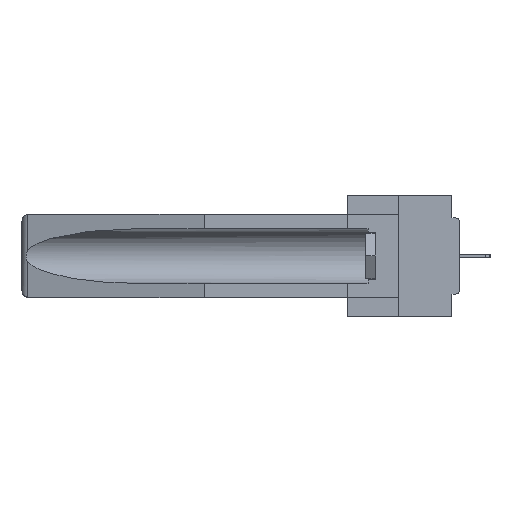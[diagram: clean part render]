
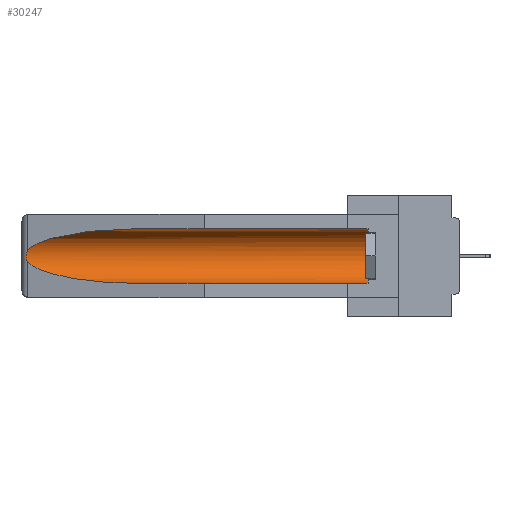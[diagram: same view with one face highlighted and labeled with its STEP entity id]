
A CAD part, left-side view. The second image highlights one B-rep face of the part: STEP entity #30247.
In plain terms, the highlighted cylindrical face has radius 2.857 mm (diameter 5.715 mm), a partial arc.
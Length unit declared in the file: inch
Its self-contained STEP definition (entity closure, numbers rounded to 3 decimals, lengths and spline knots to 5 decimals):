
#1117 = FACE_OUTER_BOUND ( 'NONE', #20640, .T. ) ;
#1626 = LINE ( 'NONE', #13462, #16823 ) ;
#1661 = CARTESIAN_POINT ( 'NONE',  ( 0.155, 1.07973, -0.284 ) ) ;
#2852 = CARTESIAN_POINT ( 'NONE',  ( 0.26597, 1.52961, -0.15275 ) ) ;
#3808 = EDGE_CURVE ( 'NONE', #28295, #29521, #8034, .T. ) ;
#3958 = ORIENTED_EDGE ( 'NONE', *, *, #11584, .T. ) ;
#4054 = CARTESIAN_POINT ( 'NONE',  ( 0.155, 0.126, -0.1715 ) ) ;
#4344 = VERTEX_POINT ( 'NONE', #22778 ) ;
#4686 = CARTESIAN_POINT ( 'NONE',  ( 0.155, 1.07973, -0.059 ) ) ;
#5570 = EDGE_CURVE ( 'NONE', #17161, #17601, #1626, .T. ) ;
#6491 = ORIENTED_EDGE ( 'NONE', *, *, #11716, .F. ) ;
#6703 = VECTOR ( 'NONE', #26251, 39.37008 ) ;
#6877 = CARTESIAN_POINT ( 'NONE',  ( 0.26537, 1.52718, -0.19328 ) ) ;
#7277 =( BOUNDED_CURVE ( )  B_SPLINE_CURVE ( 3, ( #10689, #28624, #8088, #26341 ),
 .UNSPECIFIED., .F., .F. ) 
 B_SPLINE_CURVE_WITH_KNOTS ( ( 4, 4 ),
 ( 0.1948, 1.5708 ),
 .UNSPECIFIED. ) 
 CURVE ( )  GEOMETRIC_REPRESENTATION_ITEM ( )  RATIONAL_B_SPLINE_CURVE ( ( 1., 0.848, 0.848, 1. ) ) 
 REPRESENTATION_ITEM ( '' )  );
#8034 = B_SPLINE_CURVE_WITH_KNOTS ( 'NONE', 3,
 ( #14870, #2852, #12246, #28824, #15017, #26208, #19475, #16701, #21770, #21601 ),
 .UNSPECIFIED., .F., .F.,
 ( 4, 2, 2, 2, 4 ),
 ( 0., 0.00029, 0.00058, 0.00087, 0.00117 ),
 .UNSPECIFIED. ) ;
#8057 = DIRECTION ( 'NONE',  ( 0., 1., 0. ) ) ;
#8088 = CARTESIAN_POINT ( 'NONE',  ( 0.21114, 1.30732, -0.284 ) ) ;
#10439 = EDGE_CURVE ( 'NONE', #29521, #12492, #7277, .T. ) ;
#10689 = CARTESIAN_POINT ( 'NONE',  ( 0.26537, 1.52718, -0.19328 ) ) ;
#10832 = DIRECTION ( 'NONE',  ( 0., -1., 0. ) ) ;
#11584 = EDGE_CURVE ( 'NONE', #4344, #17161, #13330, .T. ) ;
#11716 = EDGE_CURVE ( 'NONE', #4344, #12492, #23651, .T. ) ;
#12151 = ORIENTED_EDGE ( 'NONE', *, *, #10439, .T. ) ;
#12246 = CARTESIAN_POINT ( 'NONE',  ( 0.26654, 1.53092, -0.15636 ) ) ;
#12492 = VERTEX_POINT ( 'NONE', #1661 ) ;
#13330 = CIRCLE ( 'NONE', #18687, 0.1125 ) ;
#13462 = CARTESIAN_POINT ( 'NONE',  ( 0.155, -0.30754, -0.059 ) ) ;
#14870 = CARTESIAN_POINT ( 'NONE',  ( 0.26537, 1.52718, -0.14972 ) ) ;
#15017 = CARTESIAN_POINT ( 'NONE',  ( 0.2675, 1.53308, -0.16763 ) ) ;
#15663 = CARTESIAN_POINT ( 'NONE',  ( 0.26537, 1.52718, -0.14972 ) ) ;
#15746 = DIRECTION ( 'NONE',  ( 0., 0., 1. ) ) ;
#16701 = CARTESIAN_POINT ( 'NONE',  ( 0.26655, 1.53094, -0.18657 ) ) ;
#16823 = VECTOR ( 'NONE', #22351, 39.37008 ) ;
#17161 = VERTEX_POINT ( 'NONE', #27522 ) ;
#17254 = DIRECTION ( 'NONE',  ( 0., 0., 1. ) ) ;
#17601 = VERTEX_POINT ( 'NONE', #4686 ) ;
#18124 = CARTESIAN_POINT ( 'NONE',  ( 0.21114, 1.30732, -0.059 ) ) ;
#18189 = ORIENTED_EDGE ( 'NONE', *, *, #20314, .T. ) ;
#18687 = AXIS2_PLACEMENT_3D ( 'NONE', #4054, #10832, #15746 ) ;
#19475 = CARTESIAN_POINT ( 'NONE',  ( 0.2673, 1.53269, -0.17917 ) ) ;
#19799 = ORIENTED_EDGE ( 'NONE', *, *, #5570, .T. ) ;
#20237 = CARTESIAN_POINT ( 'NONE',  ( 0.26537, 1.52718, -0.14972 ) ) ;
#20314 = EDGE_CURVE ( 'NONE', #17601, #28295, #28079, .T. ) ;
#20640 = EDGE_LOOP ( 'NONE', ( #18189, #26591, #12151, #6491, #3958, #19799 ) ) ;
#21081 = AXIS2_PLACEMENT_3D ( 'NONE', #21692, #8057, #17254 ) ;
#21601 = CARTESIAN_POINT ( 'NONE',  ( 0.26537, 1.52718, -0.19328 ) ) ;
#21692 = CARTESIAN_POINT ( 'NONE',  ( 0.155, -0.30754, -0.1715 ) ) ;
#21770 = CARTESIAN_POINT ( 'NONE',  ( 0.26597, 1.5296, -0.19026 ) ) ;
#22351 = DIRECTION ( 'NONE',  ( 0., 1., 0. ) ) ;
#22778 = CARTESIAN_POINT ( 'NONE',  ( 0.155, 0.126, -0.284 ) ) ;
#23651 = LINE ( 'NONE', #26092, #6703 ) ;
#24632 = CYLINDRICAL_SURFACE ( 'NONE', #21081, 0.1125 ) ;
#26092 = CARTESIAN_POINT ( 'NONE',  ( 0.155, -0.30754, -0.284 ) ) ;
#26208 = CARTESIAN_POINT ( 'NONE',  ( 0.2675, 1.53308, -0.17534 ) ) ;
#26251 = DIRECTION ( 'NONE',  ( 0., 1., 0. ) ) ;
#26341 = CARTESIAN_POINT ( 'NONE',  ( 0.155, 1.07973, -0.284 ) ) ;
#26591 = ORIENTED_EDGE ( 'NONE', *, *, #3808, .T. ) ;
#27332 = CARTESIAN_POINT ( 'NONE',  ( 0.155, 1.07973, -0.059 ) ) ;
#27522 = CARTESIAN_POINT ( 'NONE',  ( 0.155, 0.126, -0.059 ) ) ;
#28079 =( BOUNDED_CURVE ( )  B_SPLINE_CURVE ( 3, ( #27332, #18124, #29787, #15663 ),
 .UNSPECIFIED., .F., .F. ) 
 B_SPLINE_CURVE_WITH_KNOTS ( ( 4, 4 ),
 ( 4.71239, 6.08839 ),
 .UNSPECIFIED. ) 
 CURVE ( )  GEOMETRIC_REPRESENTATION_ITEM ( )  RATIONAL_B_SPLINE_CURVE ( ( 1., 0.848, 0.848, 1. ) ) 
 REPRESENTATION_ITEM ( '' )  );
#28295 = VERTEX_POINT ( 'NONE', #20237 ) ;
#28624 = CARTESIAN_POINT ( 'NONE',  ( 0.25451, 1.48313, -0.24835 ) ) ;
#28824 = CARTESIAN_POINT ( 'NONE',  ( 0.2673, 1.5327, -0.16383 ) ) ;
#29521 = VERTEX_POINT ( 'NONE', #6877 ) ;
#29787 = CARTESIAN_POINT ( 'NONE',  ( 0.25451, 1.48313, -0.09465 ) ) ;
#30247 = ADVANCED_FACE ( 'NONE', ( #1117 ), #24632, .F. ) ;
